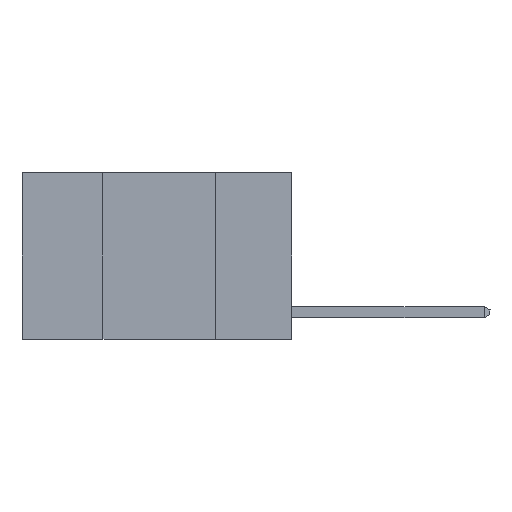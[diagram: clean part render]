
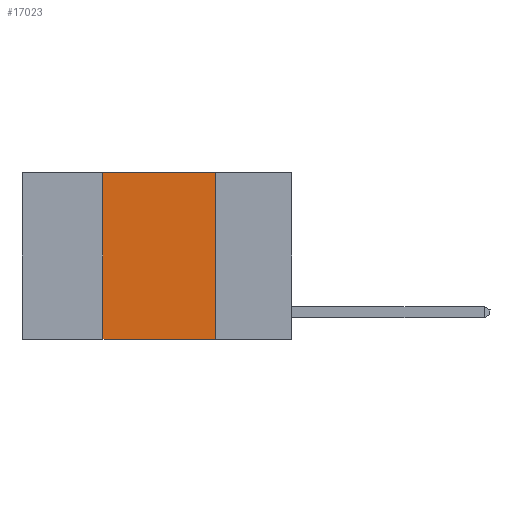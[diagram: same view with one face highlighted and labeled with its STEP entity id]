
A CAD part, left-side view. The second image highlights one B-rep face of the part: STEP entity #17023.
In plain terms, the highlighted planar face has unit normal (-1, 0, 0).
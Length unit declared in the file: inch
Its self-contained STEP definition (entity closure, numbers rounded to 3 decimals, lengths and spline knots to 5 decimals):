
#375 = ORIENTED_EDGE ( 'NONE', *, *, #14382, .T. ) ;
#518 = VERTEX_POINT ( 'NONE', #21139 ) ;
#1443 = VECTOR ( 'NONE', #9137, 39.37008 ) ;
#1640 = VERTEX_POINT ( 'NONE', #22870 ) ;
#7060 = CARTESIAN_POINT ( 'NONE',  ( 0., 0.42, 0. ) ) ;
#9137 = DIRECTION ( 'NONE',  ( 0., 0., 1. ) ) ;
#9506 = PLANE ( 'NONE',  #22864 ) ;
#9773 = LINE ( 'NONE', #22646, #19820 ) ;
#9835 = ORIENTED_EDGE ( 'NONE', *, *, #12018, .F. ) ;
#11283 = CARTESIAN_POINT ( 'NONE',  ( 0., 0.6, -0.37 ) ) ;
#11603 = DIRECTION ( 'NONE',  ( 1., 0., 0. ) ) ;
#12018 = EDGE_CURVE ( 'NONE', #19489, #19421, #22787, .T. ) ;
#13332 = DIRECTION ( 'NONE',  ( 0., -1., 0. ) ) ;
#14382 = EDGE_CURVE ( 'NONE', #19489, #518, #21708, .T. ) ;
#14559 = ORIENTED_EDGE ( 'NONE', *, *, #14896, .F. ) ;
#14896 = EDGE_CURVE ( 'NONE', #1640, #518, #9773, .T. ) ;
#15811 = CARTESIAN_POINT ( 'NONE',  ( 0., 0.42, -0.37 ) ) ;
#16415 = VECTOR ( 'NONE', #13332, 39.37008 ) ;
#16994 = EDGE_LOOP ( 'NONE', ( #14559, #25132, #9835, #375 ) ) ;
#17023 = ADVANCED_FACE ( 'NONE', ( #25582 ), #9506, .F. ) ;
#17632 = CARTESIAN_POINT ( 'NONE',  ( 0., 0.6, 0. ) ) ;
#18704 = DIRECTION ( 'NONE',  ( 0., 0., -1. ) ) ;
#19421 = VERTEX_POINT ( 'NONE', #19547 ) ;
#19429 = EDGE_CURVE ( 'NONE', #19421, #1640, #25797, .T. ) ;
#19489 = VERTEX_POINT ( 'NONE', #15811 ) ;
#19547 = CARTESIAN_POINT ( 'NONE',  ( 0., 0.42, 0. ) ) ;
#19820 = VECTOR ( 'NONE', #18704, 39.37008 ) ;
#19918 = VECTOR ( 'NONE', #25531, 39.37008 ) ;
#21139 = CARTESIAN_POINT ( 'NONE',  ( 0., 0.17, -0.37 ) ) ;
#21708 = LINE ( 'NONE', #11283, #16415 ) ;
#22646 = CARTESIAN_POINT ( 'NONE',  ( 0., 0.17, 0. ) ) ;
#22787 = LINE ( 'NONE', #7060, #1443 ) ;
#22864 = AXIS2_PLACEMENT_3D ( 'NONE', #23587, #11603, #25566 ) ;
#22870 = CARTESIAN_POINT ( 'NONE',  ( 0., 0.17, 0. ) ) ;
#23587 = CARTESIAN_POINT ( 'NONE',  ( 0., 0.6, 0. ) ) ;
#25132 = ORIENTED_EDGE ( 'NONE', *, *, #19429, .F. ) ;
#25531 = DIRECTION ( 'NONE',  ( 0., -1., 0. ) ) ;
#25566 = DIRECTION ( 'NONE',  ( 0., 0., -1. ) ) ;
#25582 = FACE_OUTER_BOUND ( 'NONE', #16994, .T. ) ;
#25797 = LINE ( 'NONE', #17632, #19918 ) ;
